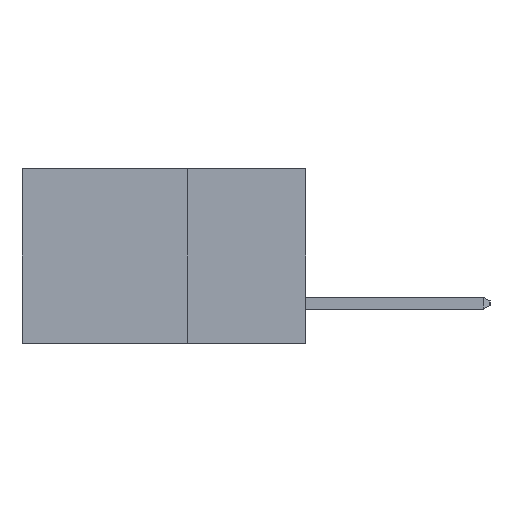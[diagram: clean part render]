
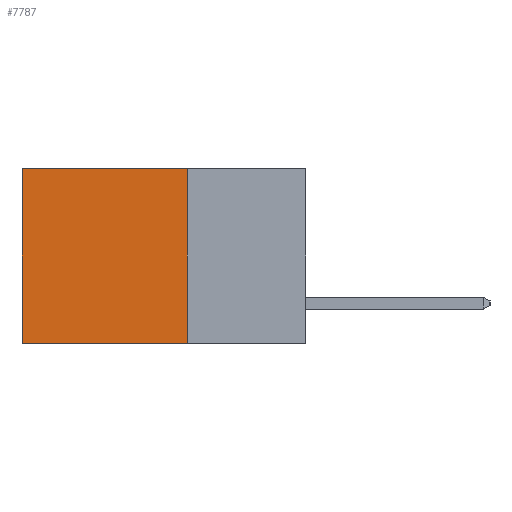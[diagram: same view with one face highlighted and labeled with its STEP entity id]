
A CAD part, left-side view. The second image highlights one B-rep face of the part: STEP entity #7787.
In plain terms, the highlighted planar face has unit normal (-1, 0, 0).
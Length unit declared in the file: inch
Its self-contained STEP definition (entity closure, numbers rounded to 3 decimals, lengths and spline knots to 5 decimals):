
#851 = CARTESIAN_POINT ( 'NONE',  ( 0.298, 0.25, -0.37 ) ) ;
#1609 = EDGE_CURVE ( 'NONE', #7087, #4795, #11073, .T. ) ;
#1646 = VECTOR ( 'NONE', #11701, 39.37008 ) ;
#1878 = DIRECTION ( 'NONE',  ( 1., 0., 0. ) ) ;
#2104 = VERTEX_POINT ( 'NONE', #4683 ) ;
#2106 = LINE ( 'NONE', #10351, #7248 ) ;
#2995 = VECTOR ( 'NONE', #9424, 39.37008 ) ;
#3016 = CARTESIAN_POINT ( 'NONE',  ( 0.298, 0.25, -0.37 ) ) ;
#3444 = EDGE_CURVE ( 'NONE', #4773, #4795, #4511, .T. ) ;
#3687 = EDGE_LOOP ( 'NONE', ( #12137, #11977, #11669, #9441 ) ) ;
#4511 = LINE ( 'NONE', #3016, #1646 ) ;
#4683 = CARTESIAN_POINT ( 'NONE',  ( 0.298, 0.25, 0. ) ) ;
#4773 = VERTEX_POINT ( 'NONE', #851 ) ;
#4795 = VERTEX_POINT ( 'NONE', #5121 ) ;
#5121 = CARTESIAN_POINT ( 'NONE',  ( 0.298, 0.6, -0.37 ) ) ;
#5123 = FACE_OUTER_BOUND ( 'NONE', #3687, .T. ) ;
#5725 = LINE ( 'NONE', #7539, #2995 ) ;
#7005 = PLANE ( 'NONE',  #9265 ) ;
#7087 = VERTEX_POINT ( 'NONE', #8620 ) ;
#7248 = VECTOR ( 'NONE', #9432, 39.37008 ) ;
#7539 = CARTESIAN_POINT ( 'NONE',  ( 0.298, 0.25, 0. ) ) ;
#7787 = ADVANCED_FACE ( 'NONE', ( #5123 ), #7005, .F. ) ;
#8124 = EDGE_CURVE ( 'NONE', #2104, #4773, #5725, .T. ) ;
#8330 = VECTOR ( 'NONE', #12290, 39.37008 ) ;
#8620 = CARTESIAN_POINT ( 'NONE',  ( 0.298, 0.6, 0. ) ) ;
#8897 = DIRECTION ( 'NONE',  ( 0., 0., -1. ) ) ;
#9265 = AXIS2_PLACEMENT_3D ( 'NONE', #11610, #1878, #8897 ) ;
#9382 = CARTESIAN_POINT ( 'NONE',  ( 0.298, 0.6, 0. ) ) ;
#9424 = DIRECTION ( 'NONE',  ( 0., 0., -1. ) ) ;
#9432 = DIRECTION ( 'NONE',  ( 0., 1., 0. ) ) ;
#9441 = ORIENTED_EDGE ( 'NONE', *, *, #10925, .T. ) ;
#10351 = CARTESIAN_POINT ( 'NONE',  ( 0.298, 0.25, 0. ) ) ;
#10925 = EDGE_CURVE ( 'NONE', #2104, #7087, #2106, .T. ) ;
#11073 = LINE ( 'NONE', #9382, #8330 ) ;
#11610 = CARTESIAN_POINT ( 'NONE',  ( 0.298, 0.25, 0. ) ) ;
#11669 = ORIENTED_EDGE ( 'NONE', *, *, #8124, .F. ) ;
#11701 = DIRECTION ( 'NONE',  ( 0., 1., 0. ) ) ;
#11977 = ORIENTED_EDGE ( 'NONE', *, *, #3444, .F. ) ;
#12137 = ORIENTED_EDGE ( 'NONE', *, *, #1609, .T. ) ;
#12290 = DIRECTION ( 'NONE',  ( 0., 0., -1. ) ) ;
